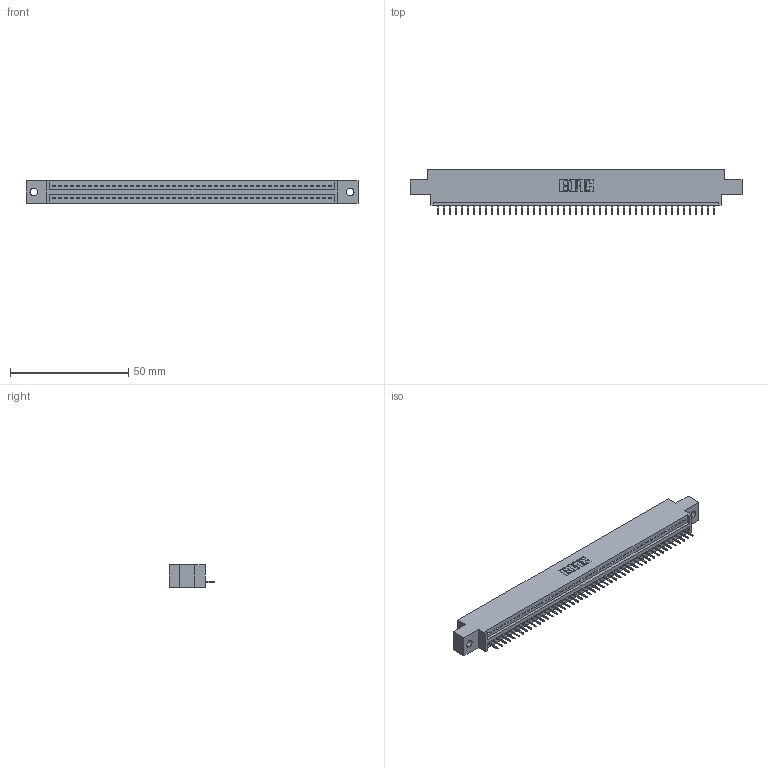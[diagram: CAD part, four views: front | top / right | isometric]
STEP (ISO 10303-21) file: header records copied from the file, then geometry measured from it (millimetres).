
FILE_DESCRIPTION (( 'STEP AP203' ), '1' );
FILE_NAME ('345-047-524-602.STEP', '2019-10-09T02:12:01', ( '' ), ( '' ), 'SwSTEP 2.0', 'SolidWorks 2016', '' );
FILE_SCHEMA (( 'CONFIG_CONTROL_DESIGN' ));
Length unit declared in the file: inch
Products named in the file (3): 345 Part_0.170 Offset - 0.128 Dia; 345-292-001_345-293-124; 345-047-524-602
Assembly tree (48 placements, depth 2):
  345-047-524-602
    345 Part_0.170 Offset - 0.128 Dia
    345-292-001_345-293-124  x47
Bounding box: 140.59 x 19.35 x 9.4 mm (x, y, z)
Volume: 13058.5 mm3; surface area: 16682.9 mm2
Topology: 48 solids, 48 shells, 3044 faces, 8813 edges, 5686 vertices
Faces by surface type: plane 2246, cylinder 798
Entity records: 34909 total; most frequent: CARTESIAN_POINT 6053, ORIENTED_EDGE 6034, DIRECTION 5279, EDGE_CURVE 3017, VECTOR 2701, LINE 2701, VERTEX_POINT 2006, AXIS2_PLACEMENT_3D 1289
